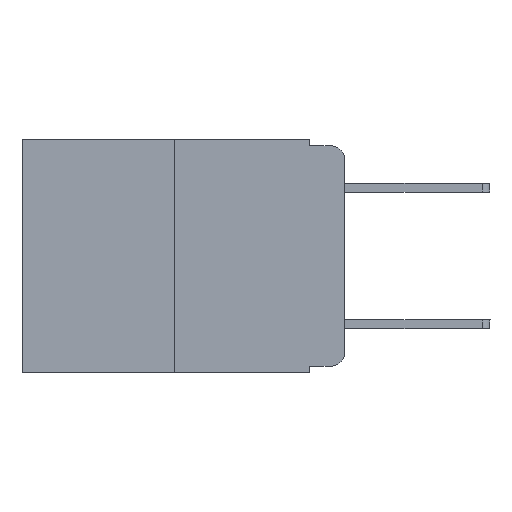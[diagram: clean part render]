
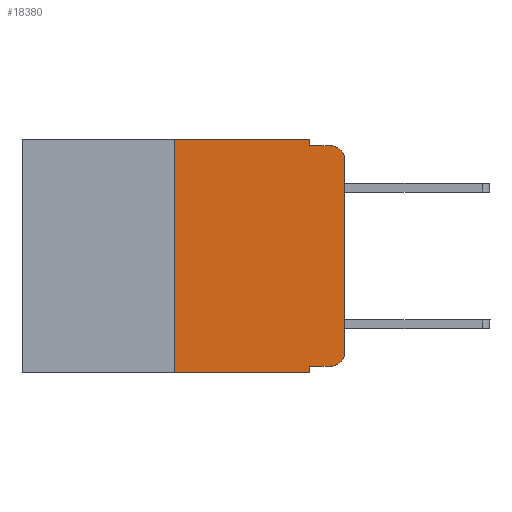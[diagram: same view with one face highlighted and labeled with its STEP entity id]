
A CAD part, left-side view. The second image highlights one B-rep face of the part: STEP entity #18380.
In plain terms, the highlighted planar face has unit normal (-1, 0, 0).
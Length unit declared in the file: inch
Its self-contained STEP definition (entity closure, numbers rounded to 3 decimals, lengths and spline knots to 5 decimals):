
#30 = ORIENTED_EDGE ( 'NONE', *, *, #2656, .F. ) ;
#81 = LINE ( 'NONE', #209, #9170 ) ;
#130 = ORIENTED_EDGE ( 'NONE', *, *, #3279, .T. ) ;
#209 = CARTESIAN_POINT ( 'NONE',  ( 0., 0.051, -0.01 ) ) ;
#510 = DIRECTION ( 'NONE',  ( 0., 0., 1. ) ) ;
#531 = CIRCLE ( 'NONE', #9338, 0.02 ) ;
#812 = LINE ( 'NONE', #12351, #16249 ) ;
#1140 = CARTESIAN_POINT ( 'NONE',  ( 0., 0., -0.313 ) ) ;
#1927 = VERTEX_POINT ( 'NONE', #4691 ) ;
#2140 = DIRECTION ( 'NONE',  ( 0., -1., 0. ) ) ;
#2347 = VERTEX_POINT ( 'NONE', #9318 ) ;
#2494 = CARTESIAN_POINT ( 'NONE',  ( 0., 0.02, -0.313 ) ) ;
#2656 = EDGE_CURVE ( 'NONE', #16039, #18442, #812, .T. ) ;
#2666 = DIRECTION ( 'NONE',  ( 0., 0., -1. ) ) ;
#3279 = EDGE_CURVE ( 'NONE', #6761, #9107, #531, .T. ) ;
#3559 = VERTEX_POINT ( 'NONE', #8280 ) ;
#3941 = EDGE_CURVE ( 'NONE', #17954, #6761, #15921, .T. ) ;
#4104 = DIRECTION ( 'NONE',  ( 0., 0., -1. ) ) ;
#4182 = CARTESIAN_POINT ( 'NONE',  ( 0., 0.02, -0.01 ) ) ;
#4691 = CARTESIAN_POINT ( 'NONE',  ( 0., 0.051, -0.333 ) ) ;
#5007 = ORIENTED_EDGE ( 'NONE', *, *, #8210, .T. ) ;
#5008 = DIRECTION ( 'NONE',  ( 0., -1., 0. ) ) ;
#5314 = CARTESIAN_POINT ( 'NONE',  ( 0., 0.473, 0. ) ) ;
#5609 = CARTESIAN_POINT ( 'NONE',  ( 0., 0.25, 0. ) ) ;
#5639 = DIRECTION ( 'NONE',  ( 0., 0., -1. ) ) ;
#5676 = DIRECTION ( 'NONE',  ( 0., 0., -1. ) ) ;
#5680 = ORIENTED_EDGE ( 'NONE', *, *, #9442, .F. ) ;
#5734 = DIRECTION ( 'NONE',  ( 0., 0., 1. ) ) ;
#5805 = CARTESIAN_POINT ( 'NONE',  ( 0., 0., 0. ) ) ;
#6761 = VERTEX_POINT ( 'NONE', #9789 ) ;
#6770 = LINE ( 'NONE', #20461, #11815 ) ;
#6849 = CIRCLE ( 'NONE', #19430, 0.02 ) ;
#7098 = CARTESIAN_POINT ( 'NONE',  ( 0., 0.051, 0. ) ) ;
#7101 = DIRECTION ( 'NONE',  ( 0., 0., -1. ) ) ;
#7500 = ORIENTED_EDGE ( 'NONE', *, *, #3941, .T. ) ;
#7621 = EDGE_CURVE ( 'NONE', #18442, #9107, #81, .T. ) ;
#7821 = VECTOR ( 'NONE', #5734, 39.37008 ) ;
#8210 = EDGE_CURVE ( 'NONE', #19154, #17954, #6849, .T. ) ;
#8280 = CARTESIAN_POINT ( 'NONE',  ( 0., 0.051, -0.343 ) ) ;
#8555 = LINE ( 'NONE', #16477, #14372 ) ;
#8812 = EDGE_CURVE ( 'NONE', #1927, #3559, #18725, .T. ) ;
#8841 = ORIENTED_EDGE ( 'NONE', *, *, #7621, .F. ) ;
#9107 = VERTEX_POINT ( 'NONE', #4182 ) ;
#9170 = VECTOR ( 'NONE', #14896, 39.37008 ) ;
#9318 = CARTESIAN_POINT ( 'NONE',  ( 0., 0.25, -0.343 ) ) ;
#9338 = AXIS2_PLACEMENT_3D ( 'NONE', #15515, #10693, #2666 ) ;
#9442 = EDGE_CURVE ( 'NONE', #14445, #16039, #19953, .T. ) ;
#9789 = CARTESIAN_POINT ( 'NONE',  ( 0., 0., -0.03 ) ) ;
#10349 = EDGE_CURVE ( 'NONE', #2347, #3559, #6770, .T. ) ;
#10693 = DIRECTION ( 'NONE',  ( -1., 0., 0. ) ) ;
#11815 = VECTOR ( 'NONE', #20527, 39.37008 ) ;
#12351 = CARTESIAN_POINT ( 'NONE',  ( 0., 0.051, 0. ) ) ;
#12501 = CARTESIAN_POINT ( 'NONE',  ( 0., 0.02, -0.333 ) ) ;
#12592 = ORIENTED_EDGE ( 'NONE', *, *, #12927, .T. ) ;
#12927 = EDGE_CURVE ( 'NONE', #1927, #19154, #18358, .T. ) ;
#13226 = CARTESIAN_POINT ( 'NONE',  ( 0., 0.051, -0.333 ) ) ;
#13379 = VECTOR ( 'NONE', #5639, 39.37008 ) ;
#13761 = DIRECTION ( 'NONE',  ( -1., 0., 0. ) ) ;
#14042 = AXIS2_PLACEMENT_3D ( 'NONE', #20036, #19909, #7101 ) ;
#14053 = VECTOR ( 'NONE', #5008, 39.37008 ) ;
#14372 = VECTOR ( 'NONE', #510, 39.37008 ) ;
#14445 = VERTEX_POINT ( 'NONE', #5609 ) ;
#14896 = DIRECTION ( 'NONE',  ( 0., -1., 0. ) ) ;
#14961 = EDGE_LOOP ( 'NONE', ( #7500, #130, #8841, #30, #5680, #19094, #17492, #16158, #12592, #5007 ) ) ;
#15515 = CARTESIAN_POINT ( 'NONE',  ( 0., 0.02, -0.03 ) ) ;
#15921 = LINE ( 'NONE', #5805, #7821 ) ;
#16039 = VERTEX_POINT ( 'NONE', #19329 ) ;
#16158 = ORIENTED_EDGE ( 'NONE', *, *, #8812, .F. ) ;
#16249 = VECTOR ( 'NONE', #5676, 39.37008 ) ;
#16477 = CARTESIAN_POINT ( 'NONE',  ( 0., 0.25, 0. ) ) ;
#16794 = PLANE ( 'NONE',  #14042 ) ;
#17438 = VECTOR ( 'NONE', #2140, 39.37008 ) ;
#17492 = ORIENTED_EDGE ( 'NONE', *, *, #10349, .T. ) ;
#17732 = EDGE_CURVE ( 'NONE', #2347, #14445, #8555, .T. ) ;
#17954 = VERTEX_POINT ( 'NONE', #1140 ) ;
#18358 = LINE ( 'NONE', #13226, #14053 ) ;
#18380 = ADVANCED_FACE ( 'NONE', ( #19651 ), #16794, .F. ) ;
#18442 = VERTEX_POINT ( 'NONE', #18638 ) ;
#18638 = CARTESIAN_POINT ( 'NONE',  ( 0., 0.051, -0.01 ) ) ;
#18725 = LINE ( 'NONE', #7098, #13379 ) ;
#19094 = ORIENTED_EDGE ( 'NONE', *, *, #17732, .F. ) ;
#19154 = VERTEX_POINT ( 'NONE', #12501 ) ;
#19329 = CARTESIAN_POINT ( 'NONE',  ( 0., 0.051, 0. ) ) ;
#19430 = AXIS2_PLACEMENT_3D ( 'NONE', #2494, #13761, #4104 ) ;
#19651 = FACE_OUTER_BOUND ( 'NONE', #14961, .T. ) ;
#19909 = DIRECTION ( 'NONE',  ( 1., 0., 0. ) ) ;
#19953 = LINE ( 'NONE', #5314, #17438 ) ;
#20036 = CARTESIAN_POINT ( 'NONE',  ( 0., 0.473, 0. ) ) ;
#20461 = CARTESIAN_POINT ( 'NONE',  ( 0., 0.473, -0.343 ) ) ;
#20527 = DIRECTION ( 'NONE',  ( 0., -1., 0. ) ) ;
